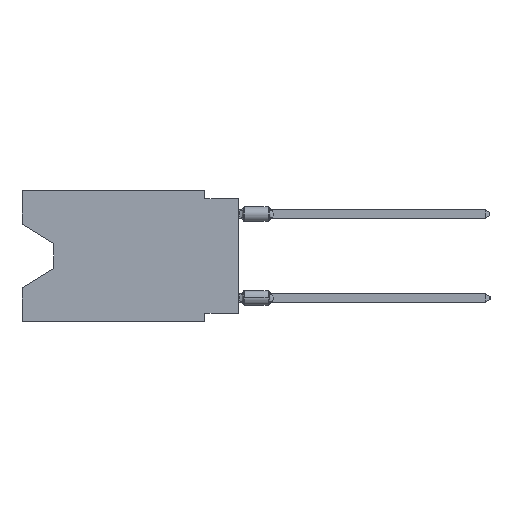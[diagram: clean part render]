
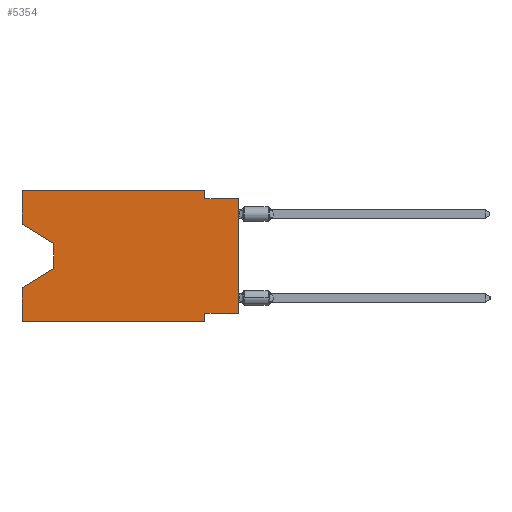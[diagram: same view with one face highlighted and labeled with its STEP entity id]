
A CAD part, left-side view. The second image highlights one B-rep face of the part: STEP entity #5354.
In plain terms, the highlighted planar face has unit normal (-1, 0, 0).
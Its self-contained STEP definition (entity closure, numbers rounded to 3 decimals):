
#466 = CARTESIAN_POINT ( 'NONE',  ( 0., 16.383, 0. ) ) ;
#968 = CARTESIAN_POINT ( 'NONE',  ( 0., 2.54, -9.906 ) ) ;
#1076 = VERTEX_POINT ( 'NONE', #17397 ) ;
#1286 = LINE ( 'NONE', #21931, #1546 ) ;
#1435 = EDGE_CURVE ( 'NONE', #4540, #14310, #11926, .T. ) ;
#1546 = VECTOR ( 'NONE', #19308, 1000. ) ;
#1954 = DIRECTION ( 'NONE',  ( 0., -1., 0. ) ) ;
#2337 = CARTESIAN_POINT ( 'NONE',  ( 0., 16.383, -9.906 ) ) ;
#2679 = VERTEX_POINT ( 'NONE', #25629 ) ;
#2731 = DIRECTION ( 'NONE',  ( 0., -1., 0. ) ) ;
#3241 = LINE ( 'NONE', #968, #3350 ) ;
#3350 = VECTOR ( 'NONE', #27704, 1000. ) ;
#3424 = CARTESIAN_POINT ( 'NONE',  ( 0., 16.383, 0. ) ) ;
#4540 = VERTEX_POINT ( 'NONE', #18833 ) ;
#5182 = CARTESIAN_POINT ( 'NONE',  ( 0., 0., -0.635 ) ) ;
#5354 = ADVANCED_FACE ( 'NONE', ( #34321 ), #31319, .F. ) ;
#5665 = AXIS2_PLACEMENT_3D ( 'NONE', #466, #6861, #12676 ) ;
#6269 = VECTOR ( 'NONE', #34658, 1000. ) ;
#6861 = DIRECTION ( 'NONE',  ( 1., 0., 0. ) ) ;
#7599 = ORIENTED_EDGE ( 'NONE', *, *, #34415, .F. ) ;
#7876 = VECTOR ( 'NONE', #22478, 1000. ) ;
#8737 = CARTESIAN_POINT ( 'NONE',  ( 0., 13.97, -4.013 ) ) ;
#9190 = CARTESIAN_POINT ( 'NONE',  ( 0., 13.97, -5.893 ) ) ;
#9305 = CARTESIAN_POINT ( 'NONE',  ( 0., 2.54, 0. ) ) ;
#9672 = VERTEX_POINT ( 'NONE', #34195 ) ;
#9748 = EDGE_CURVE ( 'NONE', #21422, #1076, #29714, .T. ) ;
#9848 = VERTEX_POINT ( 'NONE', #35517 ) ;
#10210 = DIRECTION ( 'NONE',  ( 0., 0., 1. ) ) ;
#10464 = VERTEX_POINT ( 'NONE', #38041 ) ;
#10915 = CARTESIAN_POINT ( 'NONE',  ( 0., 2.54, 0. ) ) ;
#10988 = VERTEX_POINT ( 'NONE', #10915 ) ;
#11106 = ORIENTED_EDGE ( 'NONE', *, *, #24167, .F. ) ;
#11926 = LINE ( 'NONE', #2337, #29247 ) ;
#12616 = VECTOR ( 'NONE', #19320, 1000. ) ;
#12676 = DIRECTION ( 'NONE',  ( 0., 0., -1. ) ) ;
#13003 = CARTESIAN_POINT ( 'NONE',  ( 0., 0., -0.635 ) ) ;
#13919 = DIRECTION ( 'NONE',  ( 0., 0.855, -0.519 ) ) ;
#14278 = VERTEX_POINT ( 'NONE', #9190 ) ;
#14310 = VERTEX_POINT ( 'NONE', #21425 ) ;
#14465 = VERTEX_POINT ( 'NONE', #32568 ) ;
#14774 = ORIENTED_EDGE ( 'NONE', *, *, #18818, .F. ) ;
#16348 = VECTOR ( 'NONE', #20485, 1000. ) ;
#16856 = EDGE_CURVE ( 'NONE', #9672, #14310, #3241, .T. ) ;
#17128 = ORIENTED_EDGE ( 'NONE', *, *, #28314, .T. ) ;
#17162 = LINE ( 'NONE', #29400, #27735 ) ;
#17397 = CARTESIAN_POINT ( 'NONE',  ( 0., 13.97, -4.013 ) ) ;
#17562 = LINE ( 'NONE', #8737, #23280 ) ;
#18134 = EDGE_CURVE ( 'NONE', #4540, #10464, #19852, .T. ) ;
#18437 = CARTESIAN_POINT ( 'NONE',  ( 0., 16.383, -2.546 ) ) ;
#18541 = EDGE_LOOP ( 'NONE', ( #38113, #36338, #17128, #30554, #32150, #23922, #14774, #38363, #11106, #7599, #31179, #36513 ) ) ;
#18818 = EDGE_CURVE ( 'NONE', #14465, #9672, #1286, .T. ) ;
#18833 = CARTESIAN_POINT ( 'NONE',  ( 0., 16.383, -9.906 ) ) ;
#19308 = DIRECTION ( 'NONE',  ( 0., 1., 0. ) ) ;
#19320 = DIRECTION ( 'NONE',  ( 0., 0., 1. ) ) ;
#19658 = CARTESIAN_POINT ( 'NONE',  ( 0., 16.383, 0. ) ) ;
#19852 = LINE ( 'NONE', #19658, #7876 ) ;
#20485 = DIRECTION ( 'NONE',  ( 0., -0.855, -0.519 ) ) ;
#20976 = DIRECTION ( 'NONE',  ( 0., 0., -1. ) ) ;
#21422 = VERTEX_POINT ( 'NONE', #18437 ) ;
#21425 = CARTESIAN_POINT ( 'NONE',  ( 0., 2.54, -9.906 ) ) ;
#21931 = CARTESIAN_POINT ( 'NONE',  ( 0., 0., -9.271 ) ) ;
#22478 = DIRECTION ( 'NONE',  ( 0., 0., 1. ) ) ;
#22569 = LINE ( 'NONE', #29160, #28795 ) ;
#23280 = VECTOR ( 'NONE', #20976, 1000. ) ;
#23922 = ORIENTED_EDGE ( 'NONE', *, *, #16856, .F. ) ;
#23944 = EDGE_CURVE ( 'NONE', #14465, #36309, #29138, .T. ) ;
#24167 = EDGE_CURVE ( 'NONE', #9848, #36309, #25065, .T. ) ;
#24537 = VECTOR ( 'NONE', #24965, 1000. ) ;
#24965 = DIRECTION ( 'NONE',  ( 0., 0., -1. ) ) ;
#25065 = LINE ( 'NONE', #13003, #6269 ) ;
#25629 = CARTESIAN_POINT ( 'NONE',  ( 0., 16.383, 0. ) ) ;
#27704 = DIRECTION ( 'NONE',  ( 0., 0., -1. ) ) ;
#27735 = VECTOR ( 'NONE', #1954, 1000. ) ;
#28314 = EDGE_CURVE ( 'NONE', #14278, #10464, #22569, .T. ) ;
#28355 = LINE ( 'NONE', #9305, #24537 ) ;
#28795 = VECTOR ( 'NONE', #13919, 1000. ) ;
#29138 = LINE ( 'NONE', #34558, #12616 ) ;
#29160 = CARTESIAN_POINT ( 'NONE',  ( 0., 13.97, -5.893 ) ) ;
#29247 = VECTOR ( 'NONE', #2731, 1000. ) ;
#29400 = CARTESIAN_POINT ( 'NONE',  ( 0., 16.383, 0. ) ) ;
#29714 = LINE ( 'NONE', #39127, #16348 ) ;
#30554 = ORIENTED_EDGE ( 'NONE', *, *, #18134, .F. ) ;
#31179 = ORIENTED_EDGE ( 'NONE', *, *, #36675, .F. ) ;
#31319 = PLANE ( 'NONE',  #5665 ) ;
#31661 = LINE ( 'NONE', #3424, #37293 ) ;
#32150 = ORIENTED_EDGE ( 'NONE', *, *, #1435, .T. ) ;
#32568 = CARTESIAN_POINT ( 'NONE',  ( 0., 0., -9.271 ) ) ;
#34195 = CARTESIAN_POINT ( 'NONE',  ( 0., 2.54, -9.271 ) ) ;
#34321 = FACE_OUTER_BOUND ( 'NONE', #18541, .T. ) ;
#34415 = EDGE_CURVE ( 'NONE', #10988, #9848, #28355, .T. ) ;
#34558 = CARTESIAN_POINT ( 'NONE',  ( 0., 0., 0. ) ) ;
#34658 = DIRECTION ( 'NONE',  ( 0., -1., 0. ) ) ;
#35517 = CARTESIAN_POINT ( 'NONE',  ( 0., 2.54, -0.635 ) ) ;
#36179 = EDGE_CURVE ( 'NONE', #21422, #2679, #31661, .T. ) ;
#36309 = VERTEX_POINT ( 'NONE', #5182 ) ;
#36338 = ORIENTED_EDGE ( 'NONE', *, *, #36763, .T. ) ;
#36513 = ORIENTED_EDGE ( 'NONE', *, *, #36179, .F. ) ;
#36675 = EDGE_CURVE ( 'NONE', #2679, #10988, #17162, .T. ) ;
#36763 = EDGE_CURVE ( 'NONE', #1076, #14278, #17562, .T. ) ;
#37293 = VECTOR ( 'NONE', #10210, 1000. ) ;
#38041 = CARTESIAN_POINT ( 'NONE',  ( 0., 16.383, -7.36 ) ) ;
#38113 = ORIENTED_EDGE ( 'NONE', *, *, #9748, .T. ) ;
#38363 = ORIENTED_EDGE ( 'NONE', *, *, #23944, .T. ) ;
#39127 = CARTESIAN_POINT ( 'NONE',  ( 0., 16.383, -2.546 ) ) ;
